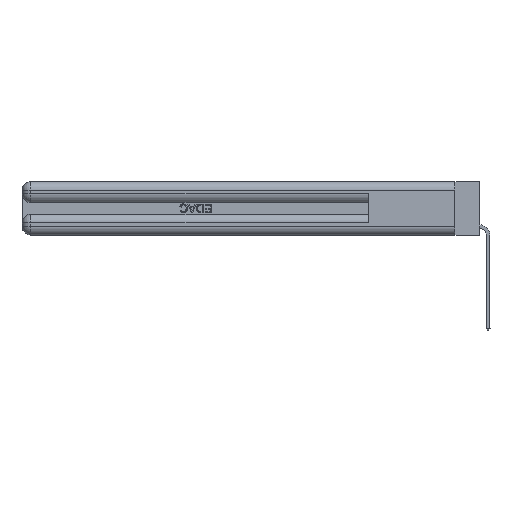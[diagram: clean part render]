
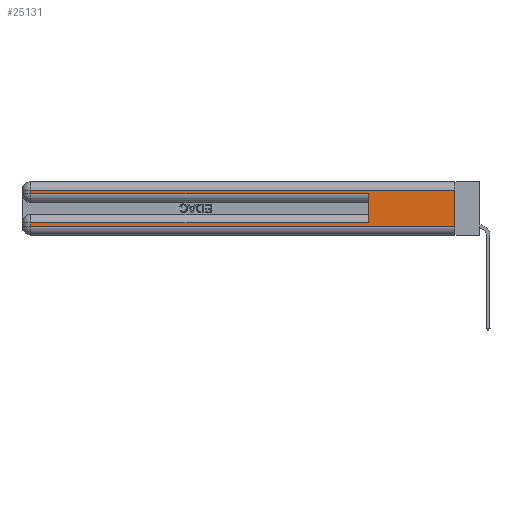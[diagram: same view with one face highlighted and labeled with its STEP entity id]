
A CAD part, left-side view. The second image highlights one B-rep face of the part: STEP entity #25131.
In plain terms, the highlighted planar face has unit normal (-1, 0, 0).
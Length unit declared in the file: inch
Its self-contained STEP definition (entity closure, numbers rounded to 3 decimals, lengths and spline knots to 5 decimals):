
#177 = CARTESIAN_POINT ( 'NONE',  ( 0., 0., 0.06 ) ) ;
#272 = VERTEX_POINT ( 'NONE', #26017 ) ;
#568 = VERTEX_POINT ( 'NONE', #7570 ) ;
#571 = DIRECTION ( 'NONE',  ( 0., 1., 0. ) ) ;
#599 = VECTOR ( 'NONE', #19468, 39.37008 ) ;
#1346 = EDGE_CURVE ( 'NONE', #14241, #272, #1404, .T. ) ;
#1404 = LINE ( 'NONE', #10093, #6541 ) ;
#1758 = CARTESIAN_POINT ( 'NONE',  ( 0., 2.94, 0.31 ) ) ;
#1789 = CARTESIAN_POINT ( 'NONE',  ( 0., 2.94, 0.37 ) ) ;
#2097 = VECTOR ( 'NONE', #2924, 39.37008 ) ;
#2264 = ORIENTED_EDGE ( 'NONE', *, *, #24114, .F. ) ;
#2430 = CARTESIAN_POINT ( 'NONE',  ( 0., 2.94, 0.085 ) ) ;
#2924 = DIRECTION ( 'NONE',  ( 0., 0., 1. ) ) ;
#4019 = ORIENTED_EDGE ( 'NONE', *, *, #28475, .T. ) ;
#5154 = LINE ( 'NONE', #18875, #20784 ) ;
#5233 = CARTESIAN_POINT ( 'NONE',  ( 0., 2.94, 0.06 ) ) ;
#5602 = DIRECTION ( 'NONE',  ( 0., 1., 0. ) ) ;
#5915 = ORIENTED_EDGE ( 'NONE', *, *, #8731, .T. ) ;
#5933 = FACE_OUTER_BOUND ( 'NONE', #9765, .T. ) ;
#6029 = VECTOR ( 'NONE', #13324, 39.37008 ) ;
#6541 = VECTOR ( 'NONE', #27783, 39.37008 ) ;
#7538 = DIRECTION ( 'NONE',  ( 0., 0., -1. ) ) ;
#7570 = CARTESIAN_POINT ( 'NONE',  ( 0., 0., 0.06 ) ) ;
#8006 = AXIS2_PLACEMENT_3D ( 'NONE', #13220, #8913, #24404 ) ;
#8333 = VECTOR ( 'NONE', #26185, 39.37008 ) ;
#8561 = ORIENTED_EDGE ( 'NONE', *, *, #21951, .T. ) ;
#8729 = ORIENTED_EDGE ( 'NONE', *, *, #20646, .T. ) ;
#8731 = EDGE_CURVE ( 'NONE', #24382, #14241, #15547, .T. ) ;
#8913 = DIRECTION ( 'NONE',  ( 1., 0., 0. ) ) ;
#9186 = ORIENTED_EDGE ( 'NONE', *, *, #9456, .T. ) ;
#9456 = EDGE_CURVE ( 'NONE', #16203, #568, #14965, .T. ) ;
#9765 = EDGE_LOOP ( 'NONE', ( #2264, #4019, #5915, #19261, #16991, #8729, #8561, #9186 ) ) ;
#10093 = CARTESIAN_POINT ( 'NONE',  ( 0., 0., 0.285 ) ) ;
#11585 = LINE ( 'NONE', #1789, #599 ) ;
#11910 = CARTESIAN_POINT ( 'NONE',  ( 0., 0., 0.37 ) ) ;
#12921 = VECTOR ( 'NONE', #571, 39.37008 ) ;
#13220 = CARTESIAN_POINT ( 'NONE',  ( 0., 0., 0.37 ) ) ;
#13324 = DIRECTION ( 'NONE',  ( 0., -1., 0. ) ) ;
#13584 = CARTESIAN_POINT ( 'NONE',  ( 0., 0.6, 0.085 ) ) ;
#13735 = LINE ( 'NONE', #13761, #2097 ) ;
#13761 = CARTESIAN_POINT ( 'NONE',  ( 0., 0.6, 0.145 ) ) ;
#14063 = VERTEX_POINT ( 'NONE', #27480 ) ;
#14241 = VERTEX_POINT ( 'NONE', #19316 ) ;
#14269 = LINE ( 'NONE', #11910, #18850 ) ;
#14965 = LINE ( 'NONE', #177, #6029 ) ;
#15547 = LINE ( 'NONE', #17410, #8333 ) ;
#16203 = VERTEX_POINT ( 'NONE', #5233 ) ;
#16991 = ORIENTED_EDGE ( 'NONE', *, *, #20468, .F. ) ;
#17410 = CARTESIAN_POINT ( 'NONE',  ( 0., 2.94, 0.37 ) ) ;
#18850 = VECTOR ( 'NONE', #7538, 39.37008 ) ;
#18875 = CARTESIAN_POINT ( 'NONE',  ( 0., 0., 0.085 ) ) ;
#19261 = ORIENTED_EDGE ( 'NONE', *, *, #1346, .T. ) ;
#19316 = CARTESIAN_POINT ( 'NONE',  ( 0., 2.94, 0.285 ) ) ;
#19468 = DIRECTION ( 'NONE',  ( 0., 0., -1. ) ) ;
#20468 = EDGE_CURVE ( 'NONE', #25240, #272, #13735, .T. ) ;
#20646 = EDGE_CURVE ( 'NONE', #25240, #28446, #5154, .T. ) ;
#20784 = VECTOR ( 'NONE', #5602, 39.37008 ) ;
#21951 = EDGE_CURVE ( 'NONE', #28446, #16203, #11585, .T. ) ;
#22229 = PLANE ( 'NONE',  #8006 ) ;
#22354 = CARTESIAN_POINT ( 'NONE',  ( 0., 0., 0.31 ) ) ;
#24114 = EDGE_CURVE ( 'NONE', #14063, #568, #14269, .T. ) ;
#24382 = VERTEX_POINT ( 'NONE', #1758 ) ;
#24404 = DIRECTION ( 'NONE',  ( 0., 0., -1. ) ) ;
#25131 = ADVANCED_FACE ( 'NONE', ( #5933 ), #22229, .F. ) ;
#25240 = VERTEX_POINT ( 'NONE', #13584 ) ;
#25420 = LINE ( 'NONE', #22354, #12921 ) ;
#26017 = CARTESIAN_POINT ( 'NONE',  ( 0., 0.6, 0.285 ) ) ;
#26185 = DIRECTION ( 'NONE',  ( 0., 0., -1. ) ) ;
#27480 = CARTESIAN_POINT ( 'NONE',  ( 0., 0., 0.31 ) ) ;
#27783 = DIRECTION ( 'NONE',  ( 0., -1., 0. ) ) ;
#28446 = VERTEX_POINT ( 'NONE', #2430 ) ;
#28475 = EDGE_CURVE ( 'NONE', #14063, #24382, #25420, .T. ) ;
